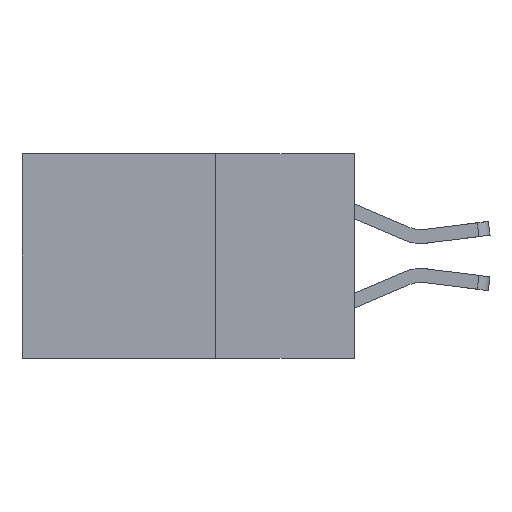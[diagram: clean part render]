
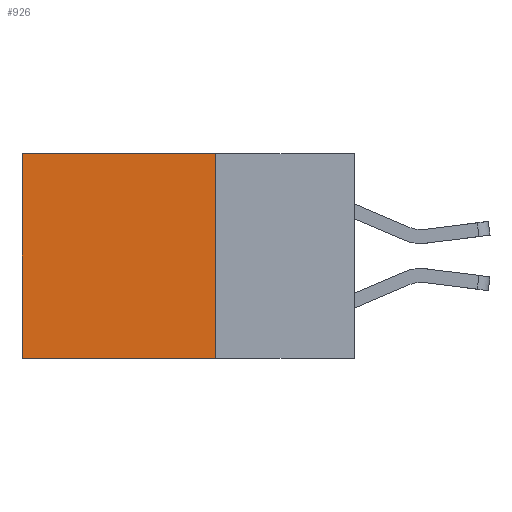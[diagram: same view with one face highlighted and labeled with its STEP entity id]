
A CAD part, left-side view. The second image highlights one B-rep face of the part: STEP entity #926.
In plain terms, the highlighted planar face has unit normal (-1, 0, 0).
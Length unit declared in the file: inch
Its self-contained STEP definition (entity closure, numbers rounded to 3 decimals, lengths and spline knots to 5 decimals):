
#772 = AXIS2_PLACEMENT_3D ( 'NONE', #8403, #4096, #4087 ) ;
#876 = EDGE_CURVE ( 'NONE', #6854, #8260, #8328, .T. ) ;
#926 = ADVANCED_FACE ( 'NONE', ( #5777 ), #8745, .F. ) ;
#1646 = VERTEX_POINT ( 'NONE', #7076 ) ;
#2320 = DIRECTION ( 'NONE',  ( 0., 0., -1. ) ) ;
#2405 = CARTESIAN_POINT ( 'NONE',  ( 0.298, 0.6, 0. ) ) ;
#2657 = EDGE_LOOP ( 'NONE', ( #3538, #10746, #6238, #8800 ) ) ;
#3538 = ORIENTED_EDGE ( 'NONE', *, *, #5528, .T. ) ;
#4045 = EDGE_CURVE ( 'NONE', #5823, #1646, #8625, .T. ) ;
#4087 = DIRECTION ( 'NONE',  ( 0., 0., -1. ) ) ;
#4096 = DIRECTION ( 'NONE',  ( 1., 0., 0. ) ) ;
#4394 = VECTOR ( 'NONE', #4543, 39.37008 ) ;
#4543 = DIRECTION ( 'NONE',  ( 0., 1., 0. ) ) ;
#5456 = CARTESIAN_POINT ( 'NONE',  ( 0.298, 0.25, 0. ) ) ;
#5528 = EDGE_CURVE ( 'NONE', #1646, #8260, #8651, .T. ) ;
#5777 = FACE_OUTER_BOUND ( 'NONE', #2657, .T. ) ;
#5823 = VERTEX_POINT ( 'NONE', #6100 ) ;
#5894 = CARTESIAN_POINT ( 'NONE',  ( 0.298, 0.25, -0.37 ) ) ;
#5899 = DIRECTION ( 'NONE',  ( 0., 1., 0. ) ) ;
#6100 = CARTESIAN_POINT ( 'NONE',  ( 0.298, 0.25, 0. ) ) ;
#6238 = ORIENTED_EDGE ( 'NONE', *, *, #7260, .F. ) ;
#6289 = VECTOR ( 'NONE', #5899, 39.37008 ) ;
#6305 = LINE ( 'NONE', #5456, #6853 ) ;
#6853 = VECTOR ( 'NONE', #10451, 39.37008 ) ;
#6854 = VERTEX_POINT ( 'NONE', #5894 ) ;
#7076 = CARTESIAN_POINT ( 'NONE',  ( 0.298, 0.6, 0. ) ) ;
#7260 = EDGE_CURVE ( 'NONE', #5823, #6854, #6305, .T. ) ;
#8260 = VERTEX_POINT ( 'NONE', #8416 ) ;
#8284 = CARTESIAN_POINT ( 'NONE',  ( 0.298, 0.25, 0. ) ) ;
#8291 = CARTESIAN_POINT ( 'NONE',  ( 0.298, 0.25, -0.37 ) ) ;
#8328 = LINE ( 'NONE', #8291, #6289 ) ;
#8403 = CARTESIAN_POINT ( 'NONE',  ( 0.298, 0.25, 0. ) ) ;
#8416 = CARTESIAN_POINT ( 'NONE',  ( 0.298, 0.6, -0.37 ) ) ;
#8625 = LINE ( 'NONE', #8284, #4394 ) ;
#8651 = LINE ( 'NONE', #2405, #10576 ) ;
#8745 = PLANE ( 'NONE',  #772 ) ;
#8800 = ORIENTED_EDGE ( 'NONE', *, *, #4045, .T. ) ;
#10451 = DIRECTION ( 'NONE',  ( 0., 0., -1. ) ) ;
#10576 = VECTOR ( 'NONE', #2320, 39.37008 ) ;
#10746 = ORIENTED_EDGE ( 'NONE', *, *, #876, .F. ) ;
